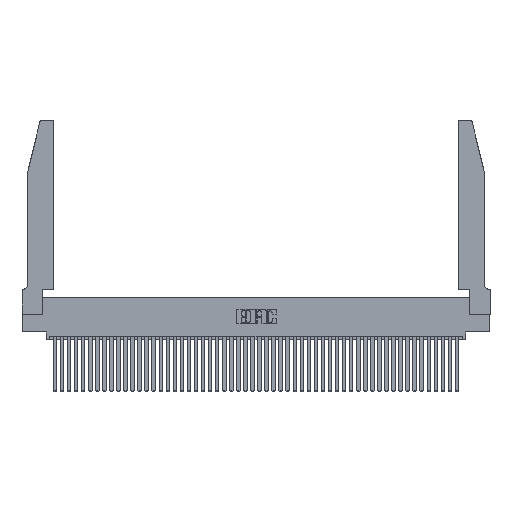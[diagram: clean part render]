
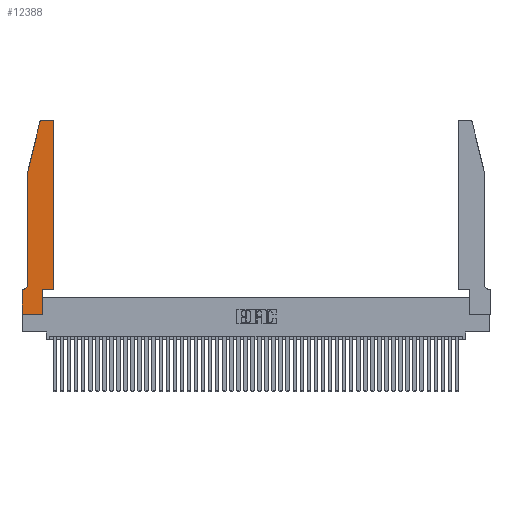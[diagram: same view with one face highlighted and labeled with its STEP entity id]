
A CAD part, top view. The second image highlights one B-rep face of the part: STEP entity #12388.
In plain terms, the highlighted planar face has unit normal (0, 0, 1).
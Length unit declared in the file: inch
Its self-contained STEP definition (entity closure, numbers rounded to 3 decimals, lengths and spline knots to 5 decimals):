
#126 = VERTEX_POINT ( 'NONE', #13738 ) ;
#4365 = EDGE_CURVE ( 'NONE', #9554, #29325, #8619, .T. ) ;
#4432 = LINE ( 'NONE', #25255, #42852 ) ;
#5089 = CARTESIAN_POINT ( 'NONE',  ( 0., 0., 0.37 ) ) ;
#5287 = EDGE_CURVE ( 'NONE', #45747, #18305, #45706, .T. ) ;
#5802 = AXIS2_PLACEMENT_3D ( 'NONE', #38614, #16353, #42301 ) ;
#6512 = CARTESIAN_POINT ( 'NONE',  ( 0.2865, 0.35, 0.37 ) ) ;
#6611 = DIRECTION ( 'NONE',  ( 1., 0., 0. ) ) ;
#7012 = EDGE_CURVE ( 'NONE', #126, #13347, #35810, .T. ) ;
#7420 = CARTESIAN_POINT ( 'NONE',  ( 0., 0., 0.37 ) ) ;
#7455 = VECTOR ( 'NONE', #23769, 39.37008 ) ;
#7830 = VECTOR ( 'NONE', #26745, 39.37008 ) ;
#7977 = FACE_OUTER_BOUND ( 'NONE', #9736, .T. ) ;
#8619 = LINE ( 'NONE', #5089, #7455 ) ;
#9172 = CARTESIAN_POINT ( 'NONE',  ( 0.0755, 2., 0.37 ) ) ;
#9554 = VERTEX_POINT ( 'NONE', #7420 ) ;
#9589 = VECTOR ( 'NONE', #21580, 39.37008 ) ;
#9736 = EDGE_LOOP ( 'NONE', ( #19451, #46757, #33275, #14207, #10136, #19994, #33739, #47196, #12847, #38482, #20793, #20918 ) ) ;
#9880 = VERTEX_POINT ( 'NONE', #13416 ) ;
#10136 = ORIENTED_EDGE ( 'NONE', *, *, #5287, .T. ) ;
#11230 = DIRECTION ( 'NONE',  ( 0., 0., 1. ) ) ;
#11506 = AXIS2_PLACEMENT_3D ( 'NONE', #18598, #11230, #37271 ) ;
#11638 = VECTOR ( 'NONE', #19659, 39.37008 ) ;
#12388 = ADVANCED_FACE ( 'NONE', ( #7977 ), #26107, .T. ) ;
#12847 = ORIENTED_EDGE ( 'NONE', *, *, #46619, .T. ) ;
#13347 = VERTEX_POINT ( 'NONE', #38654 ) ;
#13416 = CARTESIAN_POINT ( 'NONE',  ( 0.25487, 2.72718, 0.37 ) ) ;
#13738 = CARTESIAN_POINT ( 'NONE',  ( 0.4505, 2.72, 0.37 ) ) ;
#14207 = ORIENTED_EDGE ( 'NONE', *, *, #30919, .T. ) ;
#15468 = LINE ( 'NONE', #6512, #9589 ) ;
#16013 = CARTESIAN_POINT ( 'NONE',  ( 0.2865, 0.35, 0.37 ) ) ;
#16353 = DIRECTION ( 'NONE',  ( 0., 0., 1. ) ) ;
#17562 = DIRECTION ( 'NONE',  ( 0., 1., 0. ) ) ;
#17612 = DIRECTION ( 'NONE',  ( 0., 0., -1. ) ) ;
#17758 = LINE ( 'NONE', #25075, #27680 ) ;
#17941 = VERTEX_POINT ( 'NONE', #16013 ) ;
#18305 = VERTEX_POINT ( 'NONE', #43854 ) ;
#18598 = CARTESIAN_POINT ( 'NONE',  ( 0., 0.35, 0.37 ) ) ;
#19451 = ORIENTED_EDGE ( 'NONE', *, *, #26062, .T. ) ;
#19659 = DIRECTION ( 'NONE',  ( -0.239, -0.971, 0. ) ) ;
#19908 = CARTESIAN_POINT ( 'NONE',  ( 0.4205, 2.72, 0.37 ) ) ;
#19994 = ORIENTED_EDGE ( 'NONE', *, *, #46891, .T. ) ;
#20670 = EDGE_CURVE ( 'NONE', #25645, #126, #17758, .T. ) ;
#20793 = ORIENTED_EDGE ( 'NONE', *, *, #20670, .T. ) ;
#20918 = ORIENTED_EDGE ( 'NONE', *, *, #7012, .T. ) ;
#21047 = CARTESIAN_POINT ( 'NONE',  ( 0.0755, 0.42, 0.37 ) ) ;
#21580 = DIRECTION ( 'NONE',  ( 0., 1., 0. ) ) ;
#21623 = LINE ( 'NONE', #34444, #11638 ) ;
#21625 = VERTEX_POINT ( 'NONE', #30522 ) ;
#21705 = VERTEX_POINT ( 'NONE', #23545 ) ;
#21952 = CARTESIAN_POINT ( 'NONE',  ( 0.2865, 0., 0.37 ) ) ;
#23041 = CARTESIAN_POINT ( 'NONE',  ( 0.0755, 0.35, 0.37 ) ) ;
#23160 = EDGE_CURVE ( 'NONE', #9880, #21705, #21623, .T. ) ;
#23545 = CARTESIAN_POINT ( 'NONE',  ( 0.0755, 2., 0.37 ) ) ;
#23592 = CARTESIAN_POINT ( 'NONE',  ( 0.2605, 2.75, 0.37 ) ) ;
#23702 = DIRECTION ( 'NONE',  ( 1., 0., 0. ) ) ;
#23769 = DIRECTION ( 'NONE',  ( 1., 0., 0. ) ) ;
#24677 = CARTESIAN_POINT ( 'NONE',  ( 0., 0., 0.37 ) ) ;
#25075 = CARTESIAN_POINT ( 'NONE',  ( 0.4505, 0.35, 0.37 ) ) ;
#25255 = CARTESIAN_POINT ( 'NONE',  ( 0.4505, 0.35, 0.37 ) ) ;
#25645 = VERTEX_POINT ( 'NONE', #36411 ) ;
#26062 = EDGE_CURVE ( 'NONE', #13347, #41237, #37074, .T. ) ;
#26107 = PLANE ( 'NONE',  #11506 ) ;
#26745 = DIRECTION ( 'NONE',  ( -1., 0., 0. ) ) ;
#27306 = DIRECTION ( 'NONE',  ( -1., 0., 0. ) ) ;
#27680 = VECTOR ( 'NONE', #17562, 39.37008 ) ;
#27693 = LINE ( 'NONE', #23041, #7830 ) ;
#27817 = DIRECTION ( 'NONE',  ( 0., -1., 0. ) ) ;
#28388 = DIRECTION ( 'NONE',  ( 0., -1., 0. ) ) ;
#29325 = VERTEX_POINT ( 'NONE', #21952 ) ;
#29661 = EDGE_CURVE ( 'NONE', #41237, #9880, #41973, .T. ) ;
#30522 = CARTESIAN_POINT ( 'NONE',  ( 0., 0.35, 0.37 ) ) ;
#30919 = EDGE_CURVE ( 'NONE', #21705, #45747, #34330, .T. ) ;
#32296 = EDGE_CURVE ( 'NONE', #17941, #25645, #4432, .T. ) ;
#32710 = CARTESIAN_POINT ( 'NONE',  ( 0.284, 2.75, 0.37 ) ) ;
#33275 = ORIENTED_EDGE ( 'NONE', *, *, #23160, .T. ) ;
#33739 = ORIENTED_EDGE ( 'NONE', *, *, #34494, .T. ) ;
#34330 = LINE ( 'NONE', #9172, #44133 ) ;
#34444 = CARTESIAN_POINT ( 'NONE',  ( 0.0755, 2., 0.37 ) ) ;
#34494 = EDGE_CURVE ( 'NONE', #21625, #9554, #36350, .T. ) ;
#35428 = AXIS2_PLACEMENT_3D ( 'NONE', #19908, #45799, #23702 ) ;
#35810 = CIRCLE ( 'NONE', #35428, 0.03 ) ;
#35923 = VECTOR ( 'NONE', #27306, 39.37008 ) ;
#36350 = LINE ( 'NONE', #24677, #43830 ) ;
#36411 = CARTESIAN_POINT ( 'NONE',  ( 0.4505, 0.35, 0.37 ) ) ;
#37074 = LINE ( 'NONE', #23592, #35923 ) ;
#37271 = DIRECTION ( 'NONE',  ( 1., 0., 0. ) ) ;
#38482 = ORIENTED_EDGE ( 'NONE', *, *, #32296, .T. ) ;
#38614 = CARTESIAN_POINT ( 'NONE',  ( 0.284, 2.72, 0.37 ) ) ;
#38654 = CARTESIAN_POINT ( 'NONE',  ( 0.4205, 2.75, 0.37 ) ) ;
#39868 = CARTESIAN_POINT ( 'NONE',  ( 0.0055, 0.42, 0.37 ) ) ;
#41237 = VERTEX_POINT ( 'NONE', #32710 ) ;
#41973 = CIRCLE ( 'NONE', #5802, 0.03 ) ;
#42301 = DIRECTION ( 'NONE',  ( 1., 0., 0. ) ) ;
#42482 = AXIS2_PLACEMENT_3D ( 'NONE', #39868, #17612, #43556 ) ;
#42852 = VECTOR ( 'NONE', #6611, 39.37008 ) ;
#43556 = DIRECTION ( 'NONE',  ( -1., 0., 0. ) ) ;
#43830 = VECTOR ( 'NONE', #28388, 39.37008 ) ;
#43854 = CARTESIAN_POINT ( 'NONE',  ( 0.0055, 0.35, 0.37 ) ) ;
#44133 = VECTOR ( 'NONE', #27817, 39.37008 ) ;
#45706 = CIRCLE ( 'NONE', #42482, 0.07 ) ;
#45747 = VERTEX_POINT ( 'NONE', #21047 ) ;
#45799 = DIRECTION ( 'NONE',  ( 0., 0., 1. ) ) ;
#46619 = EDGE_CURVE ( 'NONE', #29325, #17941, #15468, .T. ) ;
#46757 = ORIENTED_EDGE ( 'NONE', *, *, #29661, .T. ) ;
#46891 = EDGE_CURVE ( 'NONE', #18305, #21625, #27693, .T. ) ;
#47196 = ORIENTED_EDGE ( 'NONE', *, *, #4365, .T. ) ;
